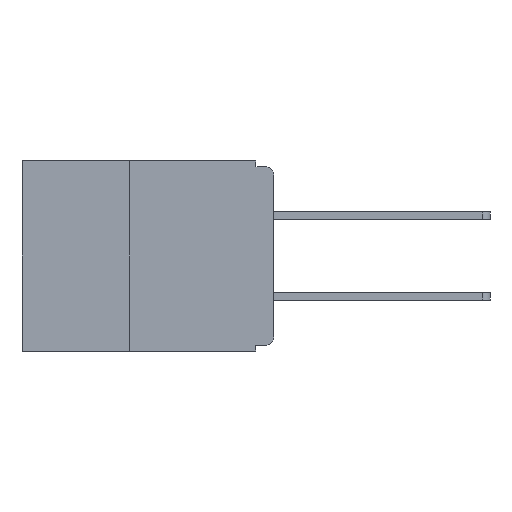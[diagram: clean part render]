
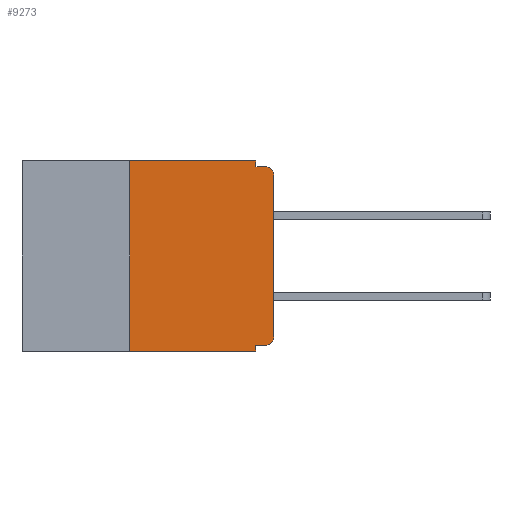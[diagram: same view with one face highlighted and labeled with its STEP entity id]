
A CAD part, left-side view. The second image highlights one B-rep face of the part: STEP entity #9273.
In plain terms, the highlighted planar face has unit normal (-1, 0, 0).
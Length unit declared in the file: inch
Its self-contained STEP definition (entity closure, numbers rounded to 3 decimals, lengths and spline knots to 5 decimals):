
#241 = EDGE_CURVE ( 'NONE', #10559, #2438, #1929, .T. ) ;
#259 = DIRECTION ( 'NONE',  ( 0., 0., -1. ) ) ;
#279 = CARTESIAN_POINT ( 'NONE',  ( 0., 0.015, -0.025 ) ) ;
#569 = ORIENTED_EDGE ( 'NONE', *, *, #25461, .T. ) ;
#979 = EDGE_CURVE ( 'NONE', #2466, #2438, #15848, .T. ) ;
#1477 = LINE ( 'NONE', #14058, #25732 ) ;
#1500 = CARTESIAN_POINT ( 'NONE',  ( 0., 0., 0. ) ) ;
#1661 = CARTESIAN_POINT ( 'NONE',  ( 0., 0.25, 0. ) ) ;
#1729 = ORIENTED_EDGE ( 'NONE', *, *, #15752, .F. ) ;
#1929 = CIRCLE ( 'NONE', #6184, 0.015 ) ;
#1949 = LINE ( 'NONE', #12276, #19971 ) ;
#2438 = VERTEX_POINT ( 'NONE', #22850 ) ;
#2466 = VERTEX_POINT ( 'NONE', #24616 ) ;
#2572 = VERTEX_POINT ( 'NONE', #22642 ) ;
#3361 = CARTESIAN_POINT ( 'NONE',  ( 0., 0.015, -0.305 ) ) ;
#3770 = VERTEX_POINT ( 'NONE', #21008 ) ;
#3977 = CARTESIAN_POINT ( 'NONE',  ( 0., 0.031, 0. ) ) ;
#4220 = CARTESIAN_POINT ( 'NONE',  ( 0., 0., -0.305 ) ) ;
#4970 = VERTEX_POINT ( 'NONE', #20411 ) ;
#5208 = ORIENTED_EDGE ( 'NONE', *, *, #21130, .T. ) ;
#5356 = EDGE_CURVE ( 'NONE', #30196, #15966, #1477, .T. ) ;
#5668 = DIRECTION ( 'NONE',  ( 0., 0., -1. ) ) ;
#5726 = DIRECTION ( 'NONE',  ( 0., 0., -1. ) ) ;
#5940 = AXIS2_PLACEMENT_3D ( 'NONE', #13288, #20370, #6294 ) ;
#6184 = AXIS2_PLACEMENT_3D ( 'NONE', #279, #26638, #259 ) ;
#6294 = DIRECTION ( 'NONE',  ( 0., 0., -1. ) ) ;
#7782 = VECTOR ( 'NONE', #5668, 39.37008 ) ;
#8127 = VECTOR ( 'NONE', #15942, 39.37008 ) ;
#8350 = VECTOR ( 'NONE', #11318, 39.37008 ) ;
#8723 = ORIENTED_EDGE ( 'NONE', *, *, #15063, .F. ) ;
#9198 = CARTESIAN_POINT ( 'NONE',  ( 0., 0., -0.025 ) ) ;
#9273 = ADVANCED_FACE ( 'NONE', ( #16362 ), #18025, .F. ) ;
#9916 = DIRECTION ( 'NONE',  ( 0., 0., -1. ) ) ;
#9967 = ORIENTED_EDGE ( 'NONE', *, *, #241, .T. ) ;
#10559 = VERTEX_POINT ( 'NONE', #9198 ) ;
#10606 = LINE ( 'NONE', #13503, #16860 ) ;
#11318 = DIRECTION ( 'NONE',  ( 0., 1., 0. ) ) ;
#12276 = CARTESIAN_POINT ( 'NONE',  ( 0., 0.031, -0.33 ) ) ;
#12973 = ORIENTED_EDGE ( 'NONE', *, *, #19016, .F. ) ;
#13288 = CARTESIAN_POINT ( 'NONE',  ( 0., 0.437, 0. ) ) ;
#13503 = CARTESIAN_POINT ( 'NONE',  ( 0., 0.437, -0.33 ) ) ;
#13989 = DIRECTION ( 'NONE',  ( 0., 0., 1. ) ) ;
#14023 = LINE ( 'NONE', #22092, #7782 ) ;
#14058 = CARTESIAN_POINT ( 'NONE',  ( 0., 0.25, -0.33 ) ) ;
#14382 = LINE ( 'NONE', #18215, #8127 ) ;
#14397 = EDGE_CURVE ( 'NONE', #3770, #23668, #14867, .T. ) ;
#14867 = CIRCLE ( 'NONE', #22093, 0.015 ) ;
#14962 = EDGE_LOOP ( 'NONE', ( #5208, #9967, #22903, #1729, #23282, #14969, #569, #8723, #12973, #17595 ) ) ;
#14969 = ORIENTED_EDGE ( 'NONE', *, *, #5356, .F. ) ;
#15063 = EDGE_CURVE ( 'NONE', #2572, #4970, #1949, .T. ) ;
#15104 = VECTOR ( 'NONE', #27949, 39.37008 ) ;
#15752 = EDGE_CURVE ( 'NONE', #16606, #2466, #14023, .T. ) ;
#15848 = LINE ( 'NONE', #16425, #15104 ) ;
#15942 = DIRECTION ( 'NONE',  ( 0., -1., 0. ) ) ;
#15966 = VERTEX_POINT ( 'NONE', #1661 ) ;
#16012 = EDGE_CURVE ( 'NONE', #15966, #16606, #14382, .T. ) ;
#16362 = FACE_OUTER_BOUND ( 'NONE', #14962, .T. ) ;
#16425 = CARTESIAN_POINT ( 'NONE',  ( 0., 0., -0.01 ) ) ;
#16606 = VERTEX_POINT ( 'NONE', #3977 ) ;
#16860 = VECTOR ( 'NONE', #29807, 39.37008 ) ;
#17595 = ORIENTED_EDGE ( 'NONE', *, *, #14397, .T. ) ;
#17949 = DIRECTION ( 'NONE',  ( 0., 0., 1. ) ) ;
#18025 = PLANE ( 'NONE',  #5940 ) ;
#18215 = CARTESIAN_POINT ( 'NONE',  ( 0., 0.437, 0. ) ) ;
#18778 = CARTESIAN_POINT ( 'NONE',  ( 0., 0.25, -0.33 ) ) ;
#19016 = EDGE_CURVE ( 'NONE', #3770, #2572, #27810, .T. ) ;
#19817 = DIRECTION ( 'NONE',  ( -1., 0., 0. ) ) ;
#19971 = VECTOR ( 'NONE', #9916, 39.37008 ) ;
#20370 = DIRECTION ( 'NONE',  ( 1., 0., 0. ) ) ;
#20411 = CARTESIAN_POINT ( 'NONE',  ( 0., 0.031, -0.33 ) ) ;
#21008 = CARTESIAN_POINT ( 'NONE',  ( 0., 0.015, -0.32 ) ) ;
#21130 = EDGE_CURVE ( 'NONE', #23668, #10559, #26993, .T. ) ;
#22093 = AXIS2_PLACEMENT_3D ( 'NONE', #3361, #19817, #5726 ) ;
#22092 = CARTESIAN_POINT ( 'NONE',  ( 0., 0.031, 0. ) ) ;
#22642 = CARTESIAN_POINT ( 'NONE',  ( 0., 0.031, -0.32 ) ) ;
#22850 = CARTESIAN_POINT ( 'NONE',  ( 0., 0.015, -0.01 ) ) ;
#22903 = ORIENTED_EDGE ( 'NONE', *, *, #979, .F. ) ;
#23024 = CARTESIAN_POINT ( 'NONE',  ( 0., 0., -0.32 ) ) ;
#23282 = ORIENTED_EDGE ( 'NONE', *, *, #16012, .F. ) ;
#23668 = VERTEX_POINT ( 'NONE', #4220 ) ;
#24616 = CARTESIAN_POINT ( 'NONE',  ( 0., 0.031, -0.01 ) ) ;
#25461 = EDGE_CURVE ( 'NONE', #30196, #4970, #10606, .T. ) ;
#25732 = VECTOR ( 'NONE', #13989, 39.37008 ) ;
#26276 = VECTOR ( 'NONE', #17949, 39.37008 ) ;
#26638 = DIRECTION ( 'NONE',  ( -1., 0., 0. ) ) ;
#26993 = LINE ( 'NONE', #1500, #26276 ) ;
#27810 = LINE ( 'NONE', #23024, #8350 ) ;
#27949 = DIRECTION ( 'NONE',  ( 0., -1., 0. ) ) ;
#29807 = DIRECTION ( 'NONE',  ( 0., -1., 0. ) ) ;
#30196 = VERTEX_POINT ( 'NONE', #18778 ) ;
